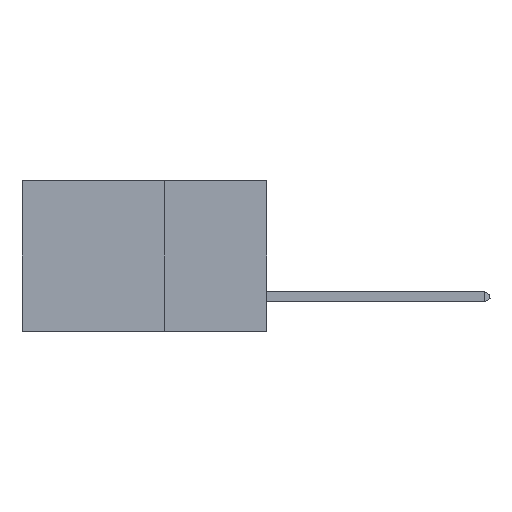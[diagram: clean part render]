
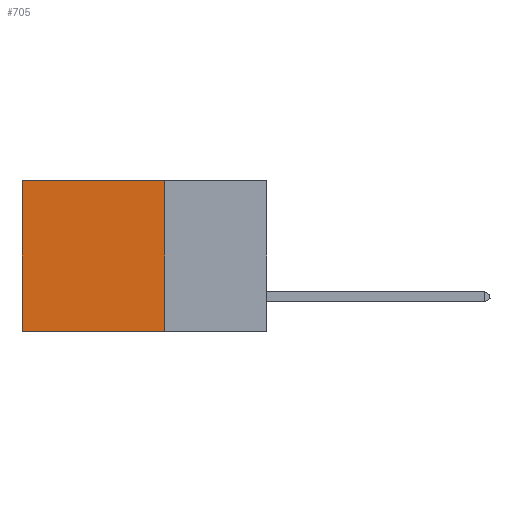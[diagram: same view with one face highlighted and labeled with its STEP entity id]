
A CAD part, left-side view. The second image highlights one B-rep face of the part: STEP entity #705.
In plain terms, the highlighted planar face has unit normal (-1, 0, 0).
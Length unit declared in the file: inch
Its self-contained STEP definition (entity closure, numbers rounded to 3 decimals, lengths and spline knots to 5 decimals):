
#57 = LINE ( 'NONE', #19996, #26693 ) ;
#457 = ORIENTED_EDGE ( 'NONE', *, *, #25641, .F. ) ;
#705 = ADVANCED_FACE ( 'NONE', ( #31340 ), #9536, .F. ) ;
#1447 = DIRECTION ( 'NONE',  ( 0., 1., 0. ) ) ;
#1473 = ORIENTED_EDGE ( 'NONE', *, *, #11434, .F. ) ;
#2359 = CARTESIAN_POINT ( 'NONE',  ( 0.2875, 0.25, 0. ) ) ;
#6056 = DIRECTION ( 'NONE',  ( 0., 0., -1. ) ) ;
#6701 = CARTESIAN_POINT ( 'NONE',  ( 0.2875, 0.6, -0.37 ) ) ;
#6875 = CARTESIAN_POINT ( 'NONE',  ( 0.2875, 0.6, 0. ) ) ;
#9536 = PLANE ( 'NONE',  #17732 ) ;
#9684 = DIRECTION ( 'NONE',  ( 0., 0., -1. ) ) ;
#10672 = VERTEX_POINT ( 'NONE', #6875 ) ;
#11434 = EDGE_CURVE ( 'NONE', #25753, #26371, #24124, .T. ) ;
#12921 = ORIENTED_EDGE ( 'NONE', *, *, #14227, .T. ) ;
#13051 = VECTOR ( 'NONE', #18578, 39.37008 ) ;
#14192 = EDGE_CURVE ( 'NONE', #25753, #10672, #16155, .T. ) ;
#14227 = EDGE_CURVE ( 'NONE', #10672, #39398, #57, .T. ) ;
#16155 = LINE ( 'NONE', #23982, #44389 ) ;
#17732 = AXIS2_PLACEMENT_3D ( 'NONE', #41870, #34611, #9684 ) ;
#18578 = DIRECTION ( 'NONE',  ( 0., 0., -1. ) ) ;
#19996 = CARTESIAN_POINT ( 'NONE',  ( 0.2875, 0.6, 0. ) ) ;
#20380 = VECTOR ( 'NONE', #1447, 39.37008 ) ;
#20646 = ORIENTED_EDGE ( 'NONE', *, *, #14192, .T. ) ;
#22323 = CARTESIAN_POINT ( 'NONE',  ( 0.2875, 0.25, -0.37 ) ) ;
#23982 = CARTESIAN_POINT ( 'NONE',  ( 0.2875, 0.25, 0. ) ) ;
#24124 = LINE ( 'NONE', #39775, #13051 ) ;
#25641 = EDGE_CURVE ( 'NONE', #26371, #39398, #27040, .T. ) ;
#25753 = VERTEX_POINT ( 'NONE', #2359 ) ;
#25913 = EDGE_LOOP ( 'NONE', ( #12921, #457, #1473, #20646 ) ) ;
#26371 = VERTEX_POINT ( 'NONE', #39234 ) ;
#26693 = VECTOR ( 'NONE', #6056, 39.37008 ) ;
#27040 = LINE ( 'NONE', #22323, #20380 ) ;
#31340 = FACE_OUTER_BOUND ( 'NONE', #25913, .T. ) ;
#34611 = DIRECTION ( 'NONE',  ( 1., 0., 0. ) ) ;
#37490 = DIRECTION ( 'NONE',  ( 0., 1., 0. ) ) ;
#39234 = CARTESIAN_POINT ( 'NONE',  ( 0.2875, 0.25, -0.37 ) ) ;
#39398 = VERTEX_POINT ( 'NONE', #6701 ) ;
#39775 = CARTESIAN_POINT ( 'NONE',  ( 0.2875, 0.25, 0. ) ) ;
#41870 = CARTESIAN_POINT ( 'NONE',  ( 0.2875, 0.25, 0. ) ) ;
#44389 = VECTOR ( 'NONE', #37490, 39.37008 ) ;
